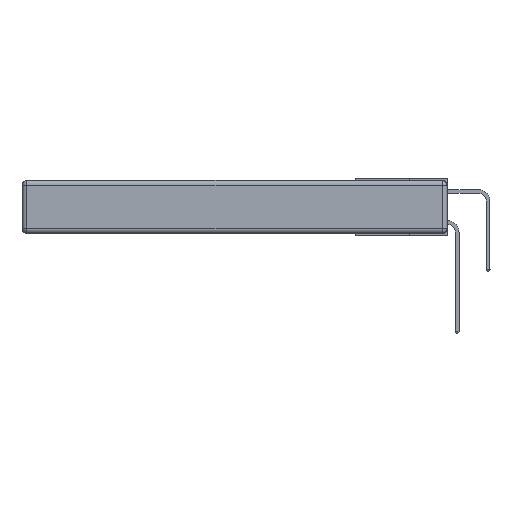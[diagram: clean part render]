
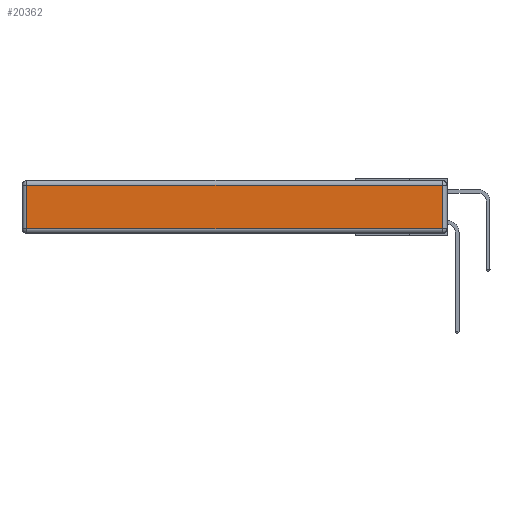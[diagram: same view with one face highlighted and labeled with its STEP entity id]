
A CAD part, left-side view. The second image highlights one B-rep face of the part: STEP entity #20362.
In plain terms, the highlighted planar face has unit normal (-1, 0, 0).
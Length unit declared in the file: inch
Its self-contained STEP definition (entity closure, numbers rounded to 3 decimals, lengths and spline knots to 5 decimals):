
#289 = LINE ( 'NONE', #417, #27780 ) ;
#417 = CARTESIAN_POINT ( 'NONE',  ( 0., 0.03, -0.343 ) ) ;
#637 = ORIENTED_EDGE ( 'NONE', *, *, #25970, .T. ) ;
#1404 = CARTESIAN_POINT ( 'NONE',  ( 0., 0.03, -0.03 ) ) ;
#2323 = CARTESIAN_POINT ( 'NONE',  ( 0., 0., -0.343 ) ) ;
#2676 = LINE ( 'NONE', #16630, #7772 ) ;
#2991 = EDGE_CURVE ( 'NONE', #3416, #5796, #14948, .T. ) ;
#3416 = VERTEX_POINT ( 'NONE', #1404 ) ;
#4182 = EDGE_LOOP ( 'NONE', ( #5576, #20964, #25448, #637 ) ) ;
#4772 = DIRECTION ( 'NONE',  ( 0., 0., 1. ) ) ;
#5576 = ORIENTED_EDGE ( 'NONE', *, *, #9657, .T. ) ;
#5796 = VERTEX_POINT ( 'NONE', #18800 ) ;
#7077 = VERTEX_POINT ( 'NONE', #21143 ) ;
#7427 = FACE_OUTER_BOUND ( 'NONE', #4182, .T. ) ;
#7772 = VECTOR ( 'NONE', #25291, 39.37008 ) ;
#8816 = VECTOR ( 'NONE', #15328, 39.37008 ) ;
#9415 = CARTESIAN_POINT ( 'NONE',  ( 0., 2.72, -0.343 ) ) ;
#9657 = EDGE_CURVE ( 'NONE', #7077, #11278, #2676, .T. ) ;
#10260 = LINE ( 'NONE', #9415, #24146 ) ;
#11278 = VERTEX_POINT ( 'NONE', #25197 ) ;
#13302 = DIRECTION ( 'NONE',  ( 0., 0., 1. ) ) ;
#13341 = AXIS2_PLACEMENT_3D ( 'NONE', #2323, #21726, #13302 ) ;
#14948 = LINE ( 'NONE', #19391, #8816 ) ;
#15328 = DIRECTION ( 'NONE',  ( 0., 1., 0. ) ) ;
#16630 = CARTESIAN_POINT ( 'NONE',  ( 0., 0., -0.313 ) ) ;
#18305 = DIRECTION ( 'NONE',  ( 0., 0., -1. ) ) ;
#18800 = CARTESIAN_POINT ( 'NONE',  ( 0., 2.72, -0.03 ) ) ;
#19391 = CARTESIAN_POINT ( 'NONE',  ( 0., 2.75, -0.03 ) ) ;
#20354 = PLANE ( 'NONE',  #13341 ) ;
#20362 = ADVANCED_FACE ( 'NONE', ( #7427 ), #20354, .T. ) ;
#20529 = EDGE_CURVE ( 'NONE', #11278, #3416, #289, .T. ) ;
#20964 = ORIENTED_EDGE ( 'NONE', *, *, #20529, .T. ) ;
#21143 = CARTESIAN_POINT ( 'NONE',  ( 0., 2.72, -0.313 ) ) ;
#21726 = DIRECTION ( 'NONE',  ( -1., 0., 0. ) ) ;
#24146 = VECTOR ( 'NONE', #18305, 39.37008 ) ;
#25197 = CARTESIAN_POINT ( 'NONE',  ( 0., 0.03, -0.313 ) ) ;
#25291 = DIRECTION ( 'NONE',  ( 0., -1., 0. ) ) ;
#25448 = ORIENTED_EDGE ( 'NONE', *, *, #2991, .T. ) ;
#25970 = EDGE_CURVE ( 'NONE', #5796, #7077, #10260, .T. ) ;
#27780 = VECTOR ( 'NONE', #4772, 39.37008 ) ;
